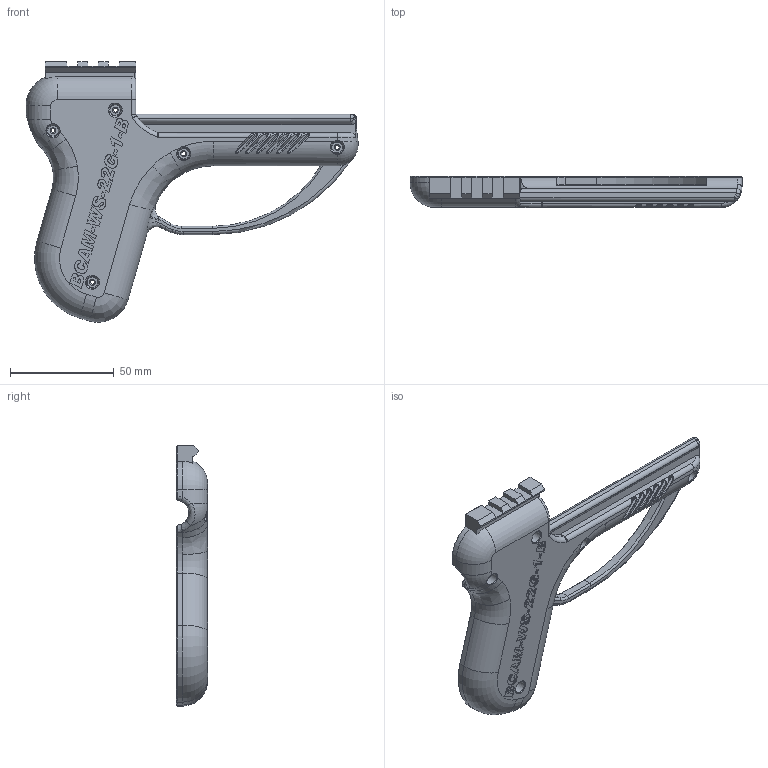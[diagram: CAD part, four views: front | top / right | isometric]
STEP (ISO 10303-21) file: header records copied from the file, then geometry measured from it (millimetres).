
FILE_DESCRIPTION(('FreeCAD Model'),'2;1');
FILE_NAME('Open CASCADE Shape Model','2022-12-07T11:24:41',('Author'),( ''),'Open CASCADE STEP processor 7.6','FreeCAD','Unknown');
FILE_SCHEMA(('AUTOMOTIVE_DESIGN { 1 0 10303 214 1 1 1 1 }'));
Length unit declared in the file: millimetre
Products named in the file (1): Frame-Right-Pic
Bounding box: 160 x 15 x 125.44 mm (x, y, z)
Volume: 91202.7 mm3; surface area: 26673.3 mm2
Topology: 1 solids, 1 shells, 584 faces, 1501 edges, 938 vertices
Faces by surface type: plane 246, extrusion 122, bspline 81, cylinder 75, cone 40, torus 16, revolution 4
Full cylindrical faces by diameter (mm): 2 x5, 6 x5
Entity records: 55597 total; most frequent: CARTESIAN_POINT 28683, DIRECTION 3839, ORIENTED_EDGE 2998, PCURVE 2998, DEFINITIONAL_REPRESENTATION 2998, VECTOR 2644, LINE 2522, B_SPLINE_CURVE_WITH_KNOTS 1646
